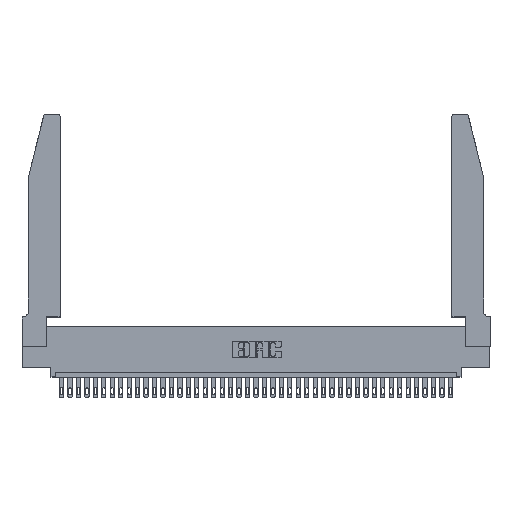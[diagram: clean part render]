
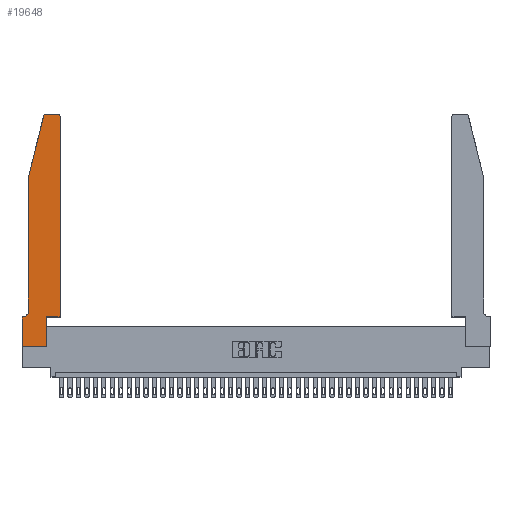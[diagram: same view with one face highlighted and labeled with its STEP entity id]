
A CAD part, top view. The second image highlights one B-rep face of the part: STEP entity #19648.
In plain terms, the highlighted planar face has unit normal (0, 0, 1).
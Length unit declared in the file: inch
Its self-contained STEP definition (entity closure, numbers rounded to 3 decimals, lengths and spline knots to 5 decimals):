
#377 = VERTEX_POINT ( 'NONE', #36638 ) ;
#922 = CARTESIAN_POINT ( 'NONE',  ( 0.0755, 2., 0.37 ) ) ;
#978 = EDGE_CURVE ( 'NONE', #10904, #30200, #6279, .T. ) ;
#1191 = ORIENTED_EDGE ( 'NONE', *, *, #21059, .T. ) ;
#1337 = CIRCLE ( 'NONE', #29698, 0.07 ) ;
#3202 = LINE ( 'NONE', #3511, #37584 ) ;
#3312 = CARTESIAN_POINT ( 'NONE',  ( 0.284, 2.72, 0.37 ) ) ;
#3511 = CARTESIAN_POINT ( 'NONE',  ( 0.0755, 2., 0.37 ) ) ;
#3800 = PLANE ( 'NONE',  #13353 ) ;
#3932 = LINE ( 'NONE', #22946, #35556 ) ;
#5001 = EDGE_CURVE ( 'NONE', #14655, #37648, #24528, .T. ) ;
#6136 = VERTEX_POINT ( 'NONE', #12427 ) ;
#6246 = DIRECTION ( 'NONE',  ( 0., 0., 1. ) ) ;
#6279 = LINE ( 'NONE', #15992, #28272 ) ;
#7260 = LINE ( 'NONE', #24809, #38846 ) ;
#8531 = VERTEX_POINT ( 'NONE', #11175 ) ;
#9062 = VECTOR ( 'NONE', #38856, 39.37008 ) ;
#9422 = EDGE_CURVE ( 'NONE', #13941, #10904, #14907, .T. ) ;
#9447 = CIRCLE ( 'NONE', #14044, 0.03 ) ;
#9815 = CARTESIAN_POINT ( 'NONE',  ( 0.284, 2.75, 0.37 ) ) ;
#9938 = DIRECTION ( 'NONE',  ( 1., 0., 0. ) ) ;
#10763 = DIRECTION ( 'NONE',  ( 0., 0., 1. ) ) ;
#10904 = VERTEX_POINT ( 'NONE', #24038 ) ;
#11175 = CARTESIAN_POINT ( 'NONE',  ( 0.0755, 0.42, 0.37 ) ) ;
#11338 = ORIENTED_EDGE ( 'NONE', *, *, #35110, .T. ) ;
#11432 = CARTESIAN_POINT ( 'NONE',  ( 0.0755, 0.35, 0.37 ) ) ;
#12427 = CARTESIAN_POINT ( 'NONE',  ( 0.25487, 2.72718, 0.37 ) ) ;
#12931 = CARTESIAN_POINT ( 'NONE',  ( 0.2865, 0.35, 0.37 ) ) ;
#13033 = CARTESIAN_POINT ( 'NONE',  ( 0.0055, 0.42, 0.37 ) ) ;
#13353 = AXIS2_PLACEMENT_3D ( 'NONE', #28292, #28418, #9938 ) ;
#13433 = VERTEX_POINT ( 'NONE', #9815 ) ;
#13690 = DIRECTION ( 'NONE',  ( 0., 1., 0. ) ) ;
#13941 = VERTEX_POINT ( 'NONE', #19763 ) ;
#14044 = AXIS2_PLACEMENT_3D ( 'NONE', #3312, #6246, #27556 ) ;
#14142 = ORIENTED_EDGE ( 'NONE', *, *, #33673, .T. ) ;
#14655 = VERTEX_POINT ( 'NONE', #12931 ) ;
#14683 = VERTEX_POINT ( 'NONE', #922 ) ;
#14741 = VERTEX_POINT ( 'NONE', #38072 ) ;
#14907 = LINE ( 'NONE', #11432, #39154 ) ;
#15683 = VERTEX_POINT ( 'NONE', #19482 ) ;
#15992 = CARTESIAN_POINT ( 'NONE',  ( 0., 0., 0.37 ) ) ;
#16645 = VECTOR ( 'NONE', #27650, 39.37008 ) ;
#16787 = ORIENTED_EDGE ( 'NONE', *, *, #29988, .T. ) ;
#19482 = CARTESIAN_POINT ( 'NONE',  ( 0.4505, 2.72, 0.37 ) ) ;
#19589 = LINE ( 'NONE', #35828, #9062 ) ;
#19648 = ADVANCED_FACE ( 'NONE', ( #22728 ), #3800, .T. ) ;
#19763 = CARTESIAN_POINT ( 'NONE',  ( 0.0055, 0.35, 0.37 ) ) ;
#19785 = DIRECTION ( 'NONE',  ( -1., 0., 0. ) ) ;
#19822 = AXIS2_PLACEMENT_3D ( 'NONE', #35263, #10763, #31775 ) ;
#20453 = DIRECTION ( 'NONE',  ( -1., 0., 0. ) ) ;
#21059 = EDGE_CURVE ( 'NONE', #37648, #15683, #3932, .T. ) ;
#22337 = ORIENTED_EDGE ( 'NONE', *, *, #37079, .T. ) ;
#22728 = FACE_OUTER_BOUND ( 'NONE', #27268, .T. ) ;
#22867 = LINE ( 'NONE', #28140, #16645 ) ;
#22946 = CARTESIAN_POINT ( 'NONE',  ( 0.4505, 0.35, 0.37 ) ) ;
#22988 = DIRECTION ( 'NONE',  ( -1., 0., 0. ) ) ;
#24038 = CARTESIAN_POINT ( 'NONE',  ( 0., 0.35, 0.37 ) ) ;
#24528 = LINE ( 'NONE', #24939, #36484 ) ;
#24809 = CARTESIAN_POINT ( 'NONE',  ( 0.2865, 0.35, 0.37 ) ) ;
#24939 = CARTESIAN_POINT ( 'NONE',  ( 0.4505, 0.35, 0.37 ) ) ;
#24957 = LINE ( 'NONE', #37750, #33128 ) ;
#25080 = EDGE_CURVE ( 'NONE', #15683, #377, #33398, .T. ) ;
#25289 = ORIENTED_EDGE ( 'NONE', *, *, #36528, .T. ) ;
#27268 = EDGE_LOOP ( 'NONE', ( #14142, #22337, #25289, #28547, #35342, #37333, #29173, #16787, #11338, #30112, #1191, #30735 ) ) ;
#27556 = DIRECTION ( 'NONE',  ( 1., 0., 0. ) ) ;
#27650 = DIRECTION ( 'NONE',  ( 1., 0., 0. ) ) ;
#28124 = DIRECTION ( 'NONE',  ( 1., 0., 0. ) ) ;
#28140 = CARTESIAN_POINT ( 'NONE',  ( 0., 0., 0.37 ) ) ;
#28272 = VECTOR ( 'NONE', #36954, 39.37008 ) ;
#28292 = CARTESIAN_POINT ( 'NONE',  ( 0., 0.35, 0.37 ) ) ;
#28418 = DIRECTION ( 'NONE',  ( 0., 0., 1. ) ) ;
#28547 = ORIENTED_EDGE ( 'NONE', *, *, #30275, .T. ) ;
#28728 = DIRECTION ( 'NONE',  ( 0., 0., -1. ) ) ;
#28941 = DIRECTION ( 'NONE',  ( 0., -1., 0. ) ) ;
#29173 = ORIENTED_EDGE ( 'NONE', *, *, #978, .T. ) ;
#29698 = AXIS2_PLACEMENT_3D ( 'NONE', #13033, #28728, #19785 ) ;
#29988 = EDGE_CURVE ( 'NONE', #30200, #14741, #22867, .T. ) ;
#30112 = ORIENTED_EDGE ( 'NONE', *, *, #5001, .T. ) ;
#30200 = VERTEX_POINT ( 'NONE', #34004 ) ;
#30275 = EDGE_CURVE ( 'NONE', #14683, #8531, #3202, .T. ) ;
#30735 = ORIENTED_EDGE ( 'NONE', *, *, #25080, .T. ) ;
#31068 = CARTESIAN_POINT ( 'NONE',  ( 0.4505, 0.35, 0.37 ) ) ;
#31775 = DIRECTION ( 'NONE',  ( 1., 0., 0. ) ) ;
#33128 = VECTOR ( 'NONE', #22988, 39.37008 ) ;
#33398 = CIRCLE ( 'NONE', #19822, 0.03 ) ;
#33673 = EDGE_CURVE ( 'NONE', #377, #13433, #24957, .T. ) ;
#34004 = CARTESIAN_POINT ( 'NONE',  ( 0., 0., 0.37 ) ) ;
#35110 = EDGE_CURVE ( 'NONE', #14741, #14655, #7260, .T. ) ;
#35263 = CARTESIAN_POINT ( 'NONE',  ( 0.4205, 2.72, 0.37 ) ) ;
#35342 = ORIENTED_EDGE ( 'NONE', *, *, #37263, .T. ) ;
#35556 = VECTOR ( 'NONE', #37178, 39.37008 ) ;
#35828 = CARTESIAN_POINT ( 'NONE',  ( 0.0755, 2., 0.37 ) ) ;
#36484 = VECTOR ( 'NONE', #28124, 39.37008 ) ;
#36528 = EDGE_CURVE ( 'NONE', #6136, #14683, #19589, .T. ) ;
#36638 = CARTESIAN_POINT ( 'NONE',  ( 0.4205, 2.75, 0.37 ) ) ;
#36954 = DIRECTION ( 'NONE',  ( 0., -1., 0. ) ) ;
#37079 = EDGE_CURVE ( 'NONE', #13433, #6136, #9447, .T. ) ;
#37178 = DIRECTION ( 'NONE',  ( 0., 1., 0. ) ) ;
#37263 = EDGE_CURVE ( 'NONE', #8531, #13941, #1337, .T. ) ;
#37333 = ORIENTED_EDGE ( 'NONE', *, *, #9422, .T. ) ;
#37584 = VECTOR ( 'NONE', #28941, 39.37008 ) ;
#37648 = VERTEX_POINT ( 'NONE', #31068 ) ;
#37750 = CARTESIAN_POINT ( 'NONE',  ( 0.2605, 2.75, 0.37 ) ) ;
#38072 = CARTESIAN_POINT ( 'NONE',  ( 0.2865, 0., 0.37 ) ) ;
#38846 = VECTOR ( 'NONE', #13690, 39.37008 ) ;
#38856 = DIRECTION ( 'NONE',  ( -0.239, -0.971, 0. ) ) ;
#39154 = VECTOR ( 'NONE', #20453, 39.37008 ) ;
